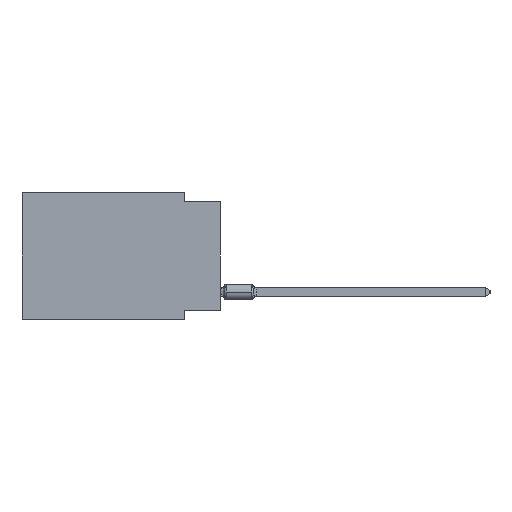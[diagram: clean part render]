
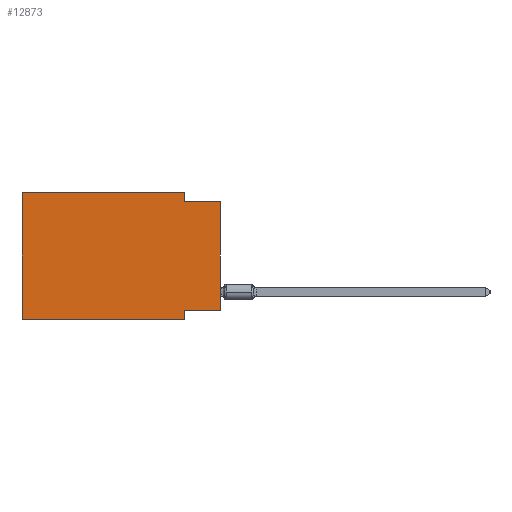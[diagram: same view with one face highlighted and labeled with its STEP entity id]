
A CAD part, left-side view. The second image highlights one B-rep face of the part: STEP entity #12873.
In plain terms, the highlighted planar face has unit normal (-1, 0, 0).
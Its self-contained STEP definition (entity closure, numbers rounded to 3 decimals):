
#421 = EDGE_CURVE ( 'NONE', #639, #16310, #17214, .T. ) ;
#516 = DIRECTION ( 'NONE',  ( 0., 0., -1. ) ) ;
#564 = CARTESIAN_POINT ( 'NONE',  ( 0., 2.54, -8.89 ) ) ;
#639 = VERTEX_POINT ( 'NONE', #4783 ) ;
#787 = EDGE_CURVE ( 'NONE', #8722, #8903, #18756, .T. ) ;
#831 = ORIENTED_EDGE ( 'NONE', *, *, #421, .F. ) ;
#1348 = VECTOR ( 'NONE', #6745, 1000. ) ;
#1574 = VECTOR ( 'NONE', #13495, 1000. ) ;
#1715 = EDGE_CURVE ( 'NONE', #7523, #8903, #16290, .T. ) ;
#2159 = CARTESIAN_POINT ( 'NONE',  ( 0., 2.54, -0.635 ) ) ;
#2260 = CARTESIAN_POINT ( 'NONE',  ( 0., 13.97, 0. ) ) ;
#2281 = CARTESIAN_POINT ( 'NONE',  ( 0., 0., -8.255 ) ) ;
#2478 = VECTOR ( 'NONE', #6829, 1000. ) ;
#3754 = LINE ( 'NONE', #2260, #2478 ) ;
#3884 = CARTESIAN_POINT ( 'NONE',  ( 0., 0., 0. ) ) ;
#4233 = DIRECTION ( 'NONE',  ( 0., 0., -1. ) ) ;
#4783 = CARTESIAN_POINT ( 'NONE',  ( 0., 13.97, 0. ) ) ;
#5060 = LINE ( 'NONE', #2281, #12029 ) ;
#5155 = CARTESIAN_POINT ( 'NONE',  ( 0., 0., -0.635 ) ) ;
#5631 = ORIENTED_EDGE ( 'NONE', *, *, #19468, .F. ) ;
#5729 = ORIENTED_EDGE ( 'NONE', *, *, #1715, .T. ) ;
#6162 = ORIENTED_EDGE ( 'NONE', *, *, #787, .F. ) ;
#6745 = DIRECTION ( 'NONE',  ( 0., -1., 0. ) ) ;
#6829 = DIRECTION ( 'NONE',  ( 0., 0., 1. ) ) ;
#7210 = CARTESIAN_POINT ( 'NONE',  ( 0., 2.54, -8.89 ) ) ;
#7464 = AXIS2_PLACEMENT_3D ( 'NONE', #13922, #9674, #15719 ) ;
#7523 = VERTEX_POINT ( 'NONE', #18990 ) ;
#8722 = VERTEX_POINT ( 'NONE', #2159 ) ;
#8761 = EDGE_CURVE ( 'NONE', #17179, #639, #3754, .T. ) ;
#8903 = VERTEX_POINT ( 'NONE', #19125 ) ;
#9665 = CARTESIAN_POINT ( 'NONE',  ( 0., 13.97, 0. ) ) ;
#9674 = DIRECTION ( 'NONE',  ( 1., 0., 0. ) ) ;
#9836 = DIRECTION ( 'NONE',  ( 0., 1., 0. ) ) ;
#11012 = LINE ( 'NONE', #11417, #15132 ) ;
#11417 = CARTESIAN_POINT ( 'NONE',  ( 0., 2.54, 0. ) ) ;
#11420 = CARTESIAN_POINT ( 'NONE',  ( 0., 13.97, -8.89 ) ) ;
#12015 = VECTOR ( 'NONE', #4233, 1000. ) ;
#12029 = VECTOR ( 'NONE', #9836, 1000. ) ;
#12426 = PLANE ( 'NONE',  #7464 ) ;
#12728 = FACE_OUTER_BOUND ( 'NONE', #14811, .T. ) ;
#12742 = VECTOR ( 'NONE', #19252, 1000. ) ;
#12873 = ADVANCED_FACE ( 'NONE', ( #12728 ), #12426, .F. ) ;
#13062 = LINE ( 'NONE', #7210, #12015 ) ;
#13308 = CARTESIAN_POINT ( 'NONE',  ( 0., 13.97, -8.89 ) ) ;
#13495 = DIRECTION ( 'NONE',  ( 0., -1., 0. ) ) ;
#13922 = CARTESIAN_POINT ( 'NONE',  ( 0., 13.97, 0. ) ) ;
#14139 = VERTEX_POINT ( 'NONE', #564 ) ;
#14695 = VERTEX_POINT ( 'NONE', #16126 ) ;
#14811 = EDGE_LOOP ( 'NONE', ( #5729, #6162, #18470, #831, #15004, #16067, #17437, #5631 ) ) ;
#14854 = EDGE_CURVE ( 'NONE', #16310, #8722, #11012, .T. ) ;
#14941 = CARTESIAN_POINT ( 'NONE',  ( 0., 2.54, 0. ) ) ;
#15004 = ORIENTED_EDGE ( 'NONE', *, *, #8761, .F. ) ;
#15132 = VECTOR ( 'NONE', #516, 1000. ) ;
#15711 = DIRECTION ( 'NONE',  ( 0., -1., 0. ) ) ;
#15719 = DIRECTION ( 'NONE',  ( 0., 0., -1. ) ) ;
#15926 = VECTOR ( 'NONE', #15711, 1000. ) ;
#16067 = ORIENTED_EDGE ( 'NONE', *, *, #19201, .T. ) ;
#16126 = CARTESIAN_POINT ( 'NONE',  ( 0., 2.54, -8.255 ) ) ;
#16290 = LINE ( 'NONE', #3884, #12742 ) ;
#16310 = VERTEX_POINT ( 'NONE', #14941 ) ;
#16503 = LINE ( 'NONE', #13308, #1574 ) ;
#17179 = VERTEX_POINT ( 'NONE', #11420 ) ;
#17214 = LINE ( 'NONE', #9665, #15926 ) ;
#17437 = ORIENTED_EDGE ( 'NONE', *, *, #17620, .F. ) ;
#17620 = EDGE_CURVE ( 'NONE', #14695, #14139, #13062, .T. ) ;
#18470 = ORIENTED_EDGE ( 'NONE', *, *, #14854, .F. ) ;
#18756 = LINE ( 'NONE', #5155, #1348 ) ;
#18990 = CARTESIAN_POINT ( 'NONE',  ( 0., 0., -8.255 ) ) ;
#19125 = CARTESIAN_POINT ( 'NONE',  ( 0., 0., -0.635 ) ) ;
#19201 = EDGE_CURVE ( 'NONE', #17179, #14139, #16503, .T. ) ;
#19252 = DIRECTION ( 'NONE',  ( 0., 0., 1. ) ) ;
#19468 = EDGE_CURVE ( 'NONE', #7523, #14695, #5060, .T. ) ;
